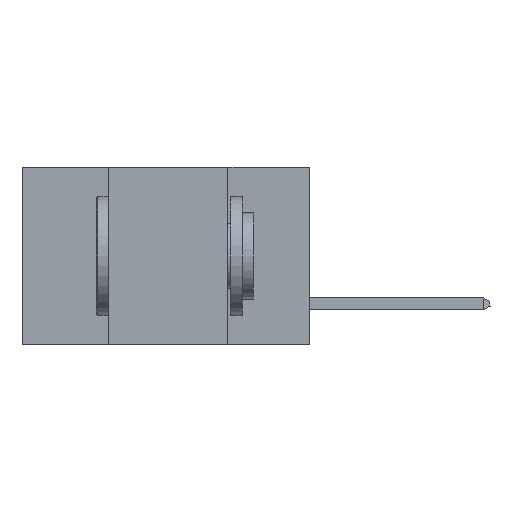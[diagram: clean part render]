
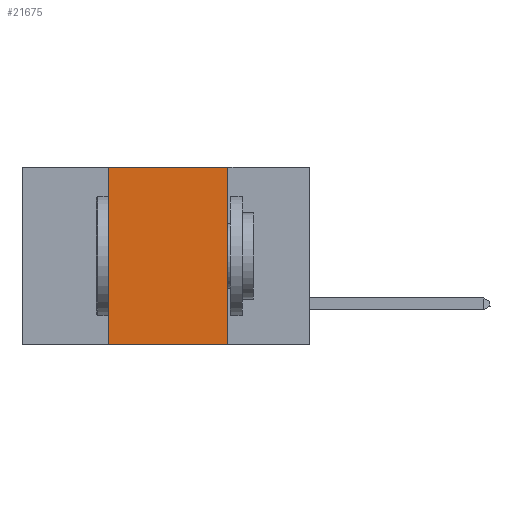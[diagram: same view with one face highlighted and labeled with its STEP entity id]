
A CAD part, left-side view. The second image highlights one B-rep face of the part: STEP entity #21675.
In plain terms, the highlighted planar face has unit normal (-1, 0, 0).
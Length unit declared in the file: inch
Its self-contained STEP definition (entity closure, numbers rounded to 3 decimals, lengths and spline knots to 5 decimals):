
#384 = PLANE ( 'NONE',  #12347 ) ;
#544 = CARTESIAN_POINT ( 'NONE',  ( 0., 0.6, 0. ) ) ;
#3113 = EDGE_CURVE ( 'NONE', #4226, #23175, #17631, .T. ) ;
#3162 = VECTOR ( 'NONE', #6505, 39.37008 ) ;
#3625 = CARTESIAN_POINT ( 'NONE',  ( 0., 0.17, -0.37 ) ) ;
#4226 = VERTEX_POINT ( 'NONE', #11369 ) ;
#4463 = VECTOR ( 'NONE', #18049, 39.37008 ) ;
#4589 = ORIENTED_EDGE ( 'NONE', *, *, #3113, .F. ) ;
#4795 = VECTOR ( 'NONE', #13609, 39.37008 ) ;
#6505 = DIRECTION ( 'NONE',  ( 0., -1., 0. ) ) ;
#6574 = VECTOR ( 'NONE', #12290, 39.37008 ) ;
#6764 = CARTESIAN_POINT ( 'NONE',  ( 0., 0.6, 0. ) ) ;
#10167 = EDGE_LOOP ( 'NONE', ( #4589, #20571, #13215, #11553 ) ) ;
#10969 = DIRECTION ( 'NONE',  ( 0., 0., -1. ) ) ;
#11369 = CARTESIAN_POINT ( 'NONE',  ( 0., 0.17, 0. ) ) ;
#11553 = ORIENTED_EDGE ( 'NONE', *, *, #26623, .T. ) ;
#12290 = DIRECTION ( 'NONE',  ( 0., 0., -1. ) ) ;
#12347 = AXIS2_PLACEMENT_3D ( 'NONE', #544, #14918, #10969 ) ;
#12359 = VERTEX_POINT ( 'NONE', #16374 ) ;
#13215 = ORIENTED_EDGE ( 'NONE', *, *, #21878, .F. ) ;
#13609 = DIRECTION ( 'NONE',  ( 0., -1., 0. ) ) ;
#14485 = CARTESIAN_POINT ( 'NONE',  ( 0., 0.42, -0.37 ) ) ;
#14918 = DIRECTION ( 'NONE',  ( 1., 0., 0. ) ) ;
#16374 = CARTESIAN_POINT ( 'NONE',  ( 0., 0.42, 0. ) ) ;
#17631 = LINE ( 'NONE', #22737, #6574 ) ;
#18049 = DIRECTION ( 'NONE',  ( 0., 0., 1. ) ) ;
#19349 = LINE ( 'NONE', #22308, #4463 ) ;
#19744 = LINE ( 'NONE', #26008, #4795 ) ;
#20571 = ORIENTED_EDGE ( 'NONE', *, *, #22153, .F. ) ;
#21623 = FACE_OUTER_BOUND ( 'NONE', #10167, .T. ) ;
#21675 = ADVANCED_FACE ( 'NONE', ( #21623 ), #384, .F. ) ;
#21878 = EDGE_CURVE ( 'NONE', #23260, #12359, #19349, .T. ) ;
#21907 = LINE ( 'NONE', #6764, #3162 ) ;
#22153 = EDGE_CURVE ( 'NONE', #12359, #4226, #21907, .T. ) ;
#22308 = CARTESIAN_POINT ( 'NONE',  ( 0., 0.42, 0. ) ) ;
#22737 = CARTESIAN_POINT ( 'NONE',  ( 0., 0.17, 0. ) ) ;
#23175 = VERTEX_POINT ( 'NONE', #3625 ) ;
#23260 = VERTEX_POINT ( 'NONE', #14485 ) ;
#26008 = CARTESIAN_POINT ( 'NONE',  ( 0., 0.6, -0.37 ) ) ;
#26623 = EDGE_CURVE ( 'NONE', #23260, #23175, #19744, .T. ) ;
